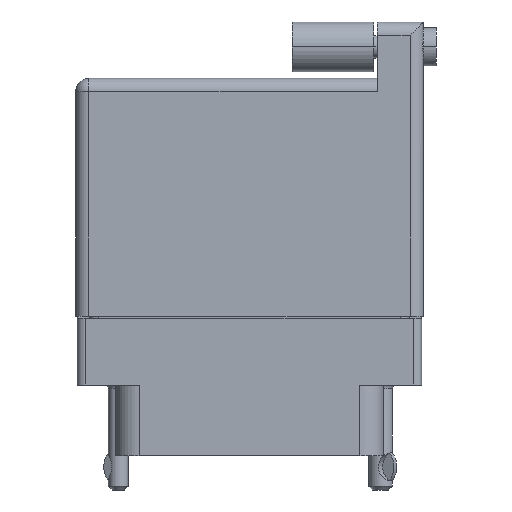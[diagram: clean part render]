
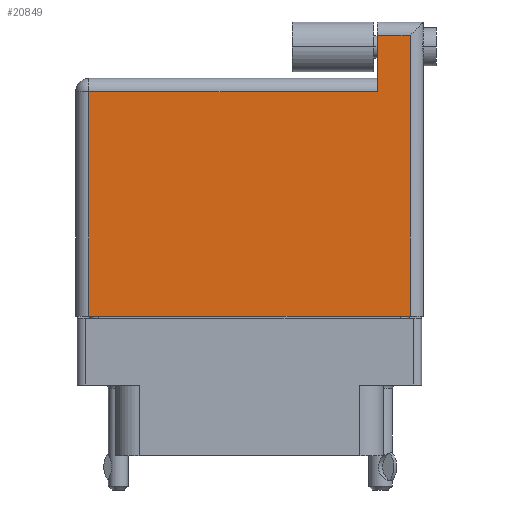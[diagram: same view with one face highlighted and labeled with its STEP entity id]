
A CAD part, front view. The second image highlights one B-rep face of the part: STEP entity #20849.
In plain terms, the highlighted face is planar.
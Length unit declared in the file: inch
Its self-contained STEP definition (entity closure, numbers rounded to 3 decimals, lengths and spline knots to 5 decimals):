
#1533 = VECTOR ( 'NONE', #30591, 39.37008 ) ;
#1982 = LINE ( 'NONE', #21134, #15290 ) ;
#2809 = CARTESIAN_POINT ( 'NONE',  ( -0.6125, -0.1, 0.3575 ) ) ;
#2929 = LINE ( 'NONE', #8772, #1533 ) ;
#3347 = CARTESIAN_POINT ( 'NONE',  ( -0.6125, -0.1, 0.3575 ) ) ;
#3514 = EDGE_CURVE ( 'NONE', #16833, #4993, #1982, .T. ) ;
#4993 = VERTEX_POINT ( 'NONE', #32437 ) ;
#7062 = VERTEX_POINT ( 'NONE', #2809 ) ;
#8064 = EDGE_CURVE ( 'NONE', #21813, #16833, #13913, .T. ) ;
#8772 = CARTESIAN_POINT ( 'NONE',  ( 0.4875, 1.02, 0.3575 ) ) ;
#10250 = DIRECTION ( 'NONE',  ( 0., 0., -1. ) ) ;
#10879 = CARTESIAN_POINT ( 'NONE',  ( 0.6125, 1.02, 0.3575 ) ) ;
#11988 = ORIENTED_EDGE ( 'NONE', *, *, #17391, .T. ) ;
#12790 = CARTESIAN_POINT ( 'NONE',  ( 0.6125, -0.1, 0.3575 ) ) ;
#12888 = PLANE ( 'NONE',  #39141 ) ;
#12967 = CARTESIAN_POINT ( 'NONE',  ( 0.4875, 0.756, 0.3575 ) ) ;
#13092 = ORIENTED_EDGE ( 'NONE', *, *, #24219, .T. ) ;
#13787 = ORIENTED_EDGE ( 'NONE', *, *, #14403, .T. ) ;
#13913 = LINE ( 'NONE', #10879, #21808 ) ;
#14403 = EDGE_CURVE ( 'NONE', #4993, #25958, #2929, .T. ) ;
#14991 = CARTESIAN_POINT ( 'NONE',  ( 0.6125, 0.97, 0.3575 ) ) ;
#15163 = LINE ( 'NONE', #25262, #32755 ) ;
#15290 = VECTOR ( 'NONE', #36104, 39.37008 ) ;
#15916 = FACE_OUTER_BOUND ( 'NONE', #39673, .T. ) ;
#16273 = DIRECTION ( 'NONE',  ( 0., -1., 0. ) ) ;
#16833 = VERTEX_POINT ( 'NONE', #14991 ) ;
#17391 = EDGE_CURVE ( 'NONE', #25958, #25541, #38759, .T. ) ;
#20484 = ORIENTED_EDGE ( 'NONE', *, *, #27305, .T. ) ;
#20849 = ADVANCED_FACE ( 'NONE', ( #15916 ), #12888, .F. ) ;
#21134 = CARTESIAN_POINT ( 'NONE',  ( -0.6625, 0.97, 0.3575 ) ) ;
#21186 = VECTOR ( 'NONE', #16273, 39.37008 ) ;
#21741 = VECTOR ( 'NONE', #39145, 39.37008 ) ;
#21808 = VECTOR ( 'NONE', #23218, 39.37008 ) ;
#21813 = VERTEX_POINT ( 'NONE', #12790 ) ;
#22154 = ORIENTED_EDGE ( 'NONE', *, *, #3514, .T. ) ;
#23218 = DIRECTION ( 'NONE',  ( 0., 1., 0. ) ) ;
#24219 = EDGE_CURVE ( 'NONE', #25541, #7062, #24950, .T. ) ;
#24950 = LINE ( 'NONE', #3347, #21186 ) ;
#25262 = CARTESIAN_POINT ( 'NONE',  ( -0.6625, -0.1, 0.3575 ) ) ;
#25336 = CARTESIAN_POINT ( 'NONE',  ( -0.6125, 0.756, 0.3575 ) ) ;
#25417 = CARTESIAN_POINT ( 'NONE',  ( -0.6625, 0.806, 0.3575 ) ) ;
#25541 = VERTEX_POINT ( 'NONE', #25336 ) ;
#25958 = VERTEX_POINT ( 'NONE', #12967 ) ;
#25972 = ORIENTED_EDGE ( 'NONE', *, *, #8064, .T. ) ;
#27305 = EDGE_CURVE ( 'NONE', #7062, #21813, #15163, .T. ) ;
#28642 = DIRECTION ( 'NONE',  ( -1., 0., 0. ) ) ;
#30591 = DIRECTION ( 'NONE',  ( 0., -1., 0. ) ) ;
#32437 = CARTESIAN_POINT ( 'NONE',  ( 0.4875, 0.97, 0.3575 ) ) ;
#32481 = CARTESIAN_POINT ( 'NONE',  ( -0.6625, 0.756, 0.3575 ) ) ;
#32755 = VECTOR ( 'NONE', #33532, 39.37008 ) ;
#33532 = DIRECTION ( 'NONE',  ( 1., 0., 0. ) ) ;
#36104 = DIRECTION ( 'NONE',  ( -1., 0., 0. ) ) ;
#38759 = LINE ( 'NONE', #32481, #21741 ) ;
#39141 = AXIS2_PLACEMENT_3D ( 'NONE', #25417, #10250, #28642 ) ;
#39145 = DIRECTION ( 'NONE',  ( -1., 0., 0. ) ) ;
#39673 = EDGE_LOOP ( 'NONE', ( #20484, #25972, #22154, #13787, #11988, #13092 ) ) ;
